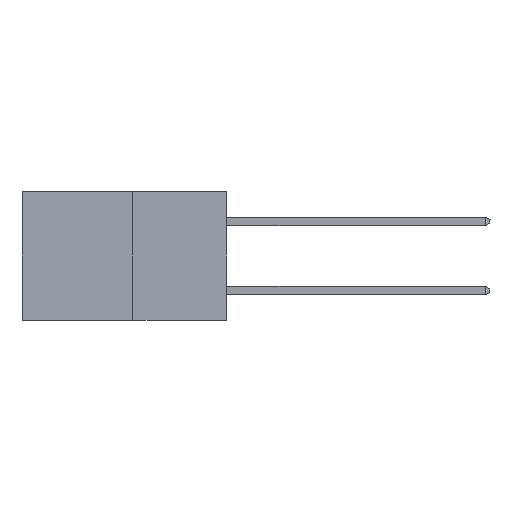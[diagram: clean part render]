
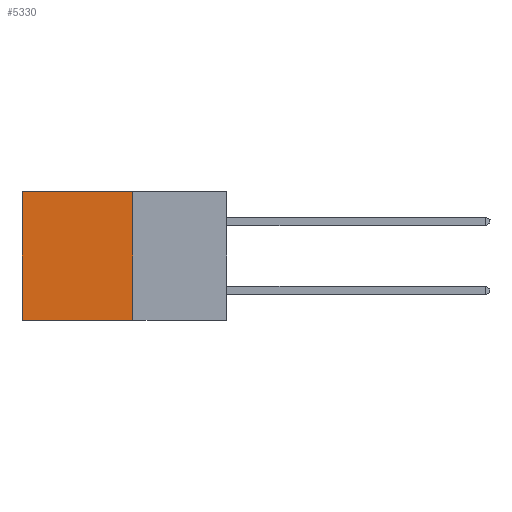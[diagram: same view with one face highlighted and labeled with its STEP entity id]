
A CAD part, left-side view. The second image highlights one B-rep face of the part: STEP entity #5330.
In plain terms, the highlighted planar face has unit normal (-1, 0, 0).
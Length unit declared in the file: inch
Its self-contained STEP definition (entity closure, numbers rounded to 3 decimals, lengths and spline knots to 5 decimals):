
#109 = ORIENTED_EDGE ( 'NONE', *, *, #5531, .T. ) ;
#2903 = VECTOR ( 'NONE', #10680, 39.37008 ) ;
#3112 = VERTEX_POINT ( 'NONE', #13920 ) ;
#3335 = CARTESIAN_POINT ( 'NONE',  ( 0.277, 0.27, -0.37 ) ) ;
#4021 = EDGE_CURVE ( 'NONE', #4387, #14167, #12420, .T. ) ;
#4387 = VERTEX_POINT ( 'NONE', #3335 ) ;
#4574 = EDGE_CURVE ( 'NONE', #3112, #4387, #14399, .T. ) ;
#5330 = ADVANCED_FACE ( 'NONE', ( #10750 ), #10988, .F. ) ;
#5360 = VECTOR ( 'NONE', #8792, 39.37008 ) ;
#5531 = EDGE_CURVE ( 'NONE', #7796, #14167, #11297, .T. ) ;
#5847 = DIRECTION ( 'NONE',  ( 0., 1., 0. ) ) ;
#5897 = CARTESIAN_POINT ( 'NONE',  ( 0.277, 0.27, 0. ) ) ;
#6336 = EDGE_CURVE ( 'NONE', #3112, #7796, #13080, .T. ) ;
#6926 = ORIENTED_EDGE ( 'NONE', *, *, #4021, .F. ) ;
#7610 = AXIS2_PLACEMENT_3D ( 'NONE', #11172, #10986, #10949 ) ;
#7796 = VERTEX_POINT ( 'NONE', #12463 ) ;
#7834 = CARTESIAN_POINT ( 'NONE',  ( 0.277, 0.27, -0.37 ) ) ;
#7868 = ORIENTED_EDGE ( 'NONE', *, *, #4574, .F. ) ;
#8205 = VECTOR ( 'NONE', #11935, 39.37008 ) ;
#8776 = CARTESIAN_POINT ( 'NONE',  ( 0.277, 0.59, -0.37 ) ) ;
#8792 = DIRECTION ( 'NONE',  ( 0., 0., -1. ) ) ;
#10680 = DIRECTION ( 'NONE',  ( 0., 1., 0. ) ) ;
#10750 = FACE_OUTER_BOUND ( 'NONE', #14892, .T. ) ;
#10816 = CARTESIAN_POINT ( 'NONE',  ( 0.277, 0.27, -0.37 ) ) ;
#10823 = CARTESIAN_POINT ( 'NONE',  ( 0.277, 0.59, -0.37 ) ) ;
#10949 = DIRECTION ( 'NONE',  ( 0., 0., -1. ) ) ;
#10986 = DIRECTION ( 'NONE',  ( 1., 0., 0. ) ) ;
#10988 = PLANE ( 'NONE',  #7610 ) ;
#11172 = CARTESIAN_POINT ( 'NONE',  ( 0.277, 0.27, -0.37 ) ) ;
#11297 = LINE ( 'NONE', #8776, #5360 ) ;
#11935 = DIRECTION ( 'NONE',  ( 0., 0., -1. ) ) ;
#12420 = LINE ( 'NONE', #10816, #2903 ) ;
#12463 = CARTESIAN_POINT ( 'NONE',  ( 0.277, 0.59, 0. ) ) ;
#12709 = VECTOR ( 'NONE', #5847, 39.37008 ) ;
#13080 = LINE ( 'NONE', #5897, #12709 ) ;
#13524 = ORIENTED_EDGE ( 'NONE', *, *, #6336, .T. ) ;
#13920 = CARTESIAN_POINT ( 'NONE',  ( 0.277, 0.27, 0. ) ) ;
#14167 = VERTEX_POINT ( 'NONE', #10823 ) ;
#14399 = LINE ( 'NONE', #7834, #8205 ) ;
#14892 = EDGE_LOOP ( 'NONE', ( #109, #6926, #7868, #13524 ) ) ;
